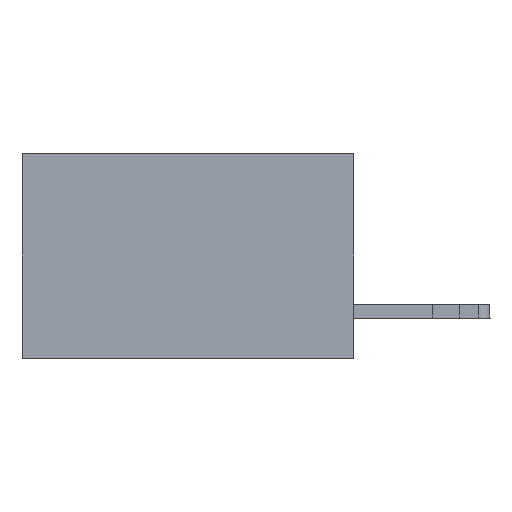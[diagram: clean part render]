
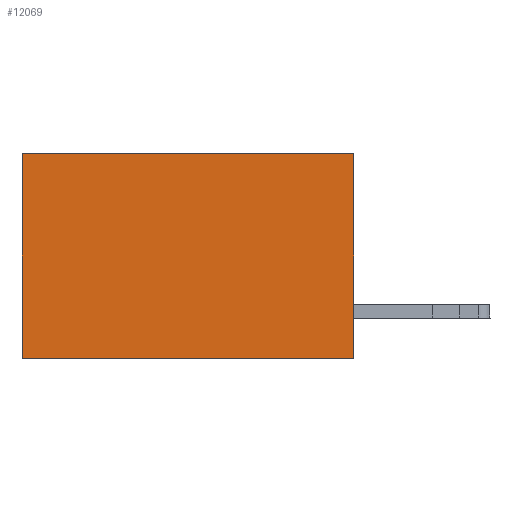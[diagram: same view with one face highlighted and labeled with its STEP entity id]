
A CAD part, left-side view. The second image highlights one B-rep face of the part: STEP entity #12069.
In plain terms, the highlighted planar face has unit normal (-1, 0, 0).
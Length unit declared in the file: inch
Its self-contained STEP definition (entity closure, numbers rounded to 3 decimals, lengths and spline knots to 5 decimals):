
#1702 = LINE ( 'NONE', #32641, #7135 ) ;
#4557 = DIRECTION ( 'NONE',  ( 0., 0., -1. ) ) ;
#4920 = CARTESIAN_POINT ( 'NONE',  ( 0.2875, 0., 0. ) ) ;
#5816 = LINE ( 'NONE', #21597, #15716 ) ;
#7135 = VECTOR ( 'NONE', #29855, 39.37008 ) ;
#7566 = VERTEX_POINT ( 'NONE', #19391 ) ;
#8427 = DIRECTION ( 'NONE',  ( 1., 0., 0. ) ) ;
#8848 = EDGE_CURVE ( 'NONE', #27847, #24406, #1702, .T. ) ;
#10600 = ORIENTED_EDGE ( 'NONE', *, *, #28523, .T. ) ;
#10615 = ORIENTED_EDGE ( 'NONE', *, *, #15469, .T. ) ;
#12069 = ADVANCED_FACE ( 'NONE', ( #31592 ), #16710, .F. ) ;
#12122 = ORIENTED_EDGE ( 'NONE', *, *, #34403, .F. ) ;
#12824 = LINE ( 'NONE', #16277, #26346 ) ;
#13074 = LINE ( 'NONE', #35301, #30224 ) ;
#14207 = DIRECTION ( 'NONE',  ( 0., 0., -1. ) ) ;
#14750 = ORIENTED_EDGE ( 'NONE', *, *, #8848, .F. ) ;
#15469 = EDGE_CURVE ( 'NONE', #16240, #7566, #12824, .T. ) ;
#15591 = CARTESIAN_POINT ( 'NONE',  ( 0.2875, 0.6, 0. ) ) ;
#15716 = VECTOR ( 'NONE', #33265, 39.37008 ) ;
#16240 = VERTEX_POINT ( 'NONE', #15591 ) ;
#16277 = CARTESIAN_POINT ( 'NONE',  ( 0.2875, 0.6, 0. ) ) ;
#16710 = PLANE ( 'NONE',  #25118 ) ;
#17747 = DIRECTION ( 'NONE',  ( 0., 1., 0. ) ) ;
#19391 = CARTESIAN_POINT ( 'NONE',  ( 0.2875, 0.6, -0.37 ) ) ;
#20203 = CARTESIAN_POINT ( 'NONE',  ( 0.2875, 0., 0. ) ) ;
#21597 = CARTESIAN_POINT ( 'NONE',  ( 0.2875, 0., 0. ) ) ;
#24406 = VERTEX_POINT ( 'NONE', #30554 ) ;
#25118 = AXIS2_PLACEMENT_3D ( 'NONE', #20203, #8427, #14207 ) ;
#26346 = VECTOR ( 'NONE', #4557, 39.37008 ) ;
#27847 = VERTEX_POINT ( 'NONE', #4920 ) ;
#28523 = EDGE_CURVE ( 'NONE', #27847, #16240, #5816, .T. ) ;
#29855 = DIRECTION ( 'NONE',  ( 0., 0., -1. ) ) ;
#30224 = VECTOR ( 'NONE', #17747, 39.37008 ) ;
#30554 = CARTESIAN_POINT ( 'NONE',  ( 0.2875, 0., -0.37 ) ) ;
#31592 = FACE_OUTER_BOUND ( 'NONE', #33529, .T. ) ;
#32641 = CARTESIAN_POINT ( 'NONE',  ( 0.2875, 0., 0. ) ) ;
#33265 = DIRECTION ( 'NONE',  ( 0., 1., 0. ) ) ;
#33529 = EDGE_LOOP ( 'NONE', ( #10615, #12122, #14750, #10600 ) ) ;
#34403 = EDGE_CURVE ( 'NONE', #24406, #7566, #13074, .T. ) ;
#35301 = CARTESIAN_POINT ( 'NONE',  ( 0.2875, 0., -0.37 ) ) ;
